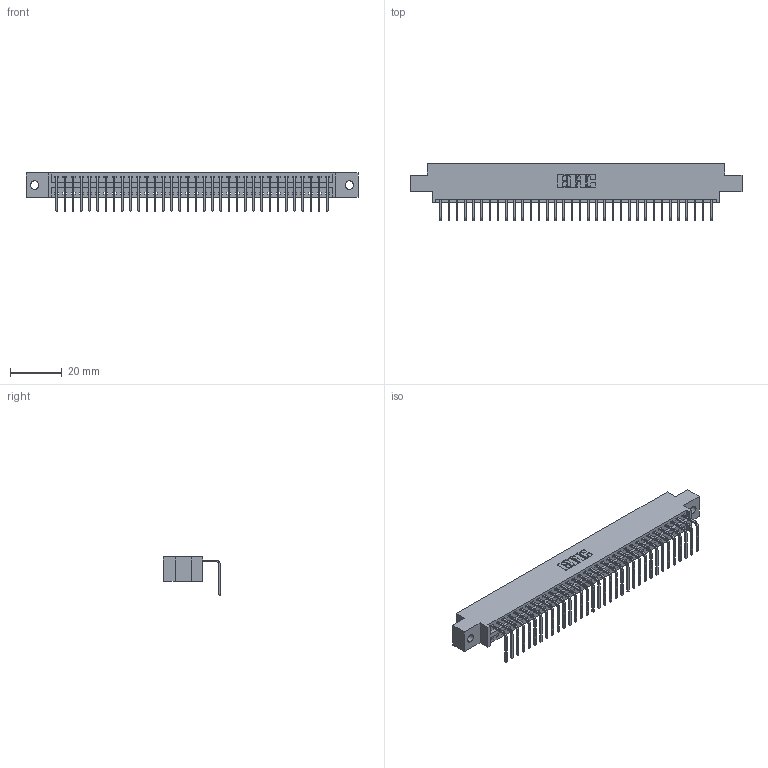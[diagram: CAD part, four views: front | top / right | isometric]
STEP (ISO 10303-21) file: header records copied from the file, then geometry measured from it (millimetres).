
FILE_DESCRIPTION (( 'STEP AP203' ), '1' );
FILE_NAME ('346-034-558-602.STEP', '2022-05-06T21:58:46', ( '' ), ( '' ), 'SwSTEP 2.0', 'SolidWorks 2020', '' );
FILE_SCHEMA (( 'CONFIG_CONTROL_DESIGN' ));
Length unit declared in the file: inch
Products named in the file (3): 346-034-558-602; 346 Part_0.170 Offset - 0.128 Dia; 345-292-001_558 Tail - 2
Assembly tree (35 placements, depth 2):
  346-034-558-602
    346 Part_0.170 Offset - 0.128 Dia
    345-292-001_558 Tail - 2  x34
Bounding box: 128.52 x 22.16 x 14.73 mm (x, y, z)
Volume: 12169.5 mm3; surface area: 15688.8 mm2
Topology: 35 solids, 35 shells, 2166 faces, 6529 edges, 4306 vertices
Faces by surface type: plane 1508, cylinder 658
Entity records: 22397 total; most frequent: CARTESIAN_POINT 3850, ORIENTED_EDGE 3818, DIRECTION 3405, EDGE_CURVE 1909, LINE 1641, VECTOR 1641, VERTEX_POINT 1270, AXIS2_PLACEMENT_3D 882
